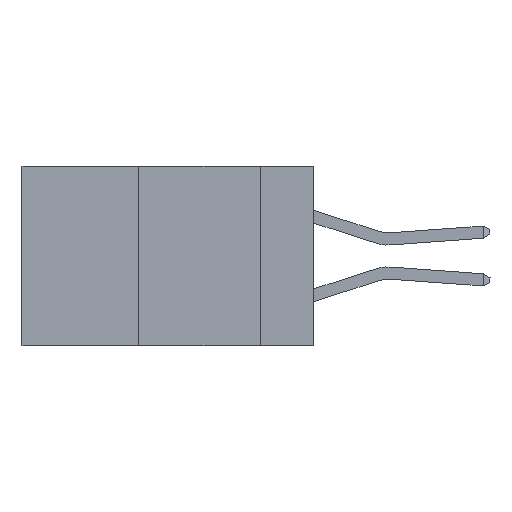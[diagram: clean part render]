
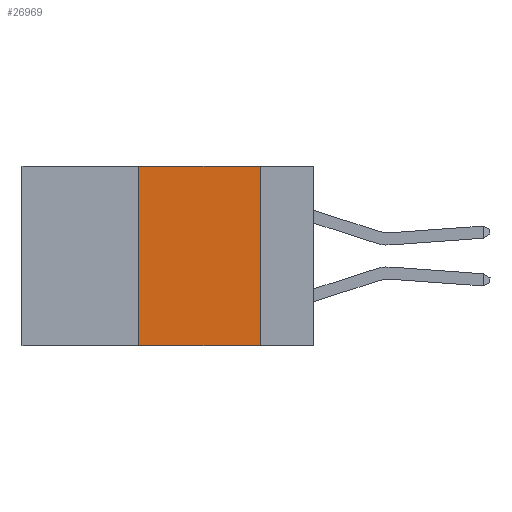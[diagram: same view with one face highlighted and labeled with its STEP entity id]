
A CAD part, left-side view. The second image highlights one B-rep face of the part: STEP entity #26969.
In plain terms, the highlighted planar face has unit normal (-1, 0, 0).
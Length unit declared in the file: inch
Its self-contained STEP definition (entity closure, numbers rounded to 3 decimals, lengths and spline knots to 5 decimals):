
#1197 = AXIS2_PLACEMENT_3D ( 'NONE', #10585, #19330, #27228 ) ;
#1325 = VECTOR ( 'NONE', #17622, 39.37008 ) ;
#1405 = CARTESIAN_POINT ( 'NONE',  ( 0., 0.36, 0. ) ) ;
#2318 = LINE ( 'NONE', #18634, #19251 ) ;
#4186 = EDGE_CURVE ( 'NONE', #9504, #29244, #8632, .T. ) ;
#4789 = EDGE_CURVE ( 'NONE', #28857, #11295, #2318, .T. ) ;
#6236 = CARTESIAN_POINT ( 'NONE',  ( 0., 0.6, 0. ) ) ;
#7152 = VECTOR ( 'NONE', #12513, 39.37008 ) ;
#7520 = ORIENTED_EDGE ( 'NONE', *, *, #22103, .F. ) ;
#8481 = CARTESIAN_POINT ( 'NONE',  ( 0., 0.11, -0.37 ) ) ;
#8632 = LINE ( 'NONE', #22284, #7152 ) ;
#9504 = VERTEX_POINT ( 'NONE', #30494 ) ;
#10418 = FACE_OUTER_BOUND ( 'NONE', #19286, .T. ) ;
#10585 = CARTESIAN_POINT ( 'NONE',  ( 0., 0.6, 0. ) ) ;
#11295 = VERTEX_POINT ( 'NONE', #1405 ) ;
#12513 = DIRECTION ( 'NONE',  ( 0., 0., -1. ) ) ;
#14102 = LINE ( 'NONE', #15992, #28223 ) ;
#15302 = PLANE ( 'NONE',  #1197 ) ;
#15992 = CARTESIAN_POINT ( 'NONE',  ( 0., 0.6, -0.37 ) ) ;
#17622 = DIRECTION ( 'NONE',  ( 0., -1., 0. ) ) ;
#18634 = CARTESIAN_POINT ( 'NONE',  ( 0., 0.36, 0. ) ) ;
#19251 = VECTOR ( 'NONE', #23316, 39.37008 ) ;
#19286 = EDGE_LOOP ( 'NONE', ( #28089, #7520, #20802, #28472 ) ) ;
#19330 = DIRECTION ( 'NONE',  ( 1., 0., 0. ) ) ;
#20802 = ORIENTED_EDGE ( 'NONE', *, *, #4789, .F. ) ;
#20873 = DIRECTION ( 'NONE',  ( 0., -1., 0. ) ) ;
#22103 = EDGE_CURVE ( 'NONE', #11295, #9504, #26408, .T. ) ;
#22284 = CARTESIAN_POINT ( 'NONE',  ( 0., 0.11, 0. ) ) ;
#23316 = DIRECTION ( 'NONE',  ( 0., 0., 1. ) ) ;
#25857 = CARTESIAN_POINT ( 'NONE',  ( 0., 0.36, -0.37 ) ) ;
#26408 = LINE ( 'NONE', #6236, #1325 ) ;
#26969 = ADVANCED_FACE ( 'NONE', ( #10418 ), #15302, .F. ) ;
#27228 = DIRECTION ( 'NONE',  ( 0., 0., -1. ) ) ;
#27924 = EDGE_CURVE ( 'NONE', #28857, #29244, #14102, .T. ) ;
#28089 = ORIENTED_EDGE ( 'NONE', *, *, #4186, .F. ) ;
#28223 = VECTOR ( 'NONE', #20873, 39.37008 ) ;
#28472 = ORIENTED_EDGE ( 'NONE', *, *, #27924, .T. ) ;
#28857 = VERTEX_POINT ( 'NONE', #25857 ) ;
#29244 = VERTEX_POINT ( 'NONE', #8481 ) ;
#30494 = CARTESIAN_POINT ( 'NONE',  ( 0., 0.11, 0. ) ) ;
